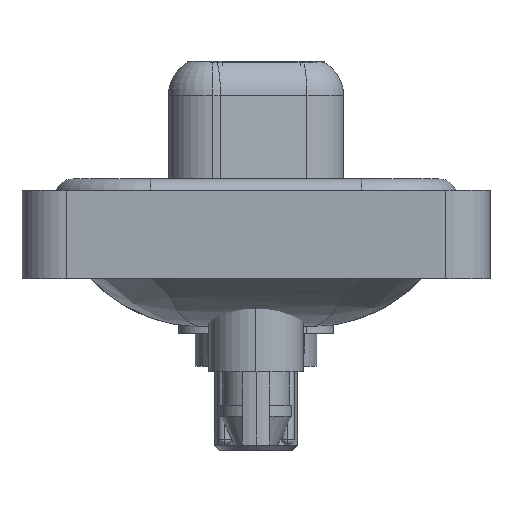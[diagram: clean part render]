
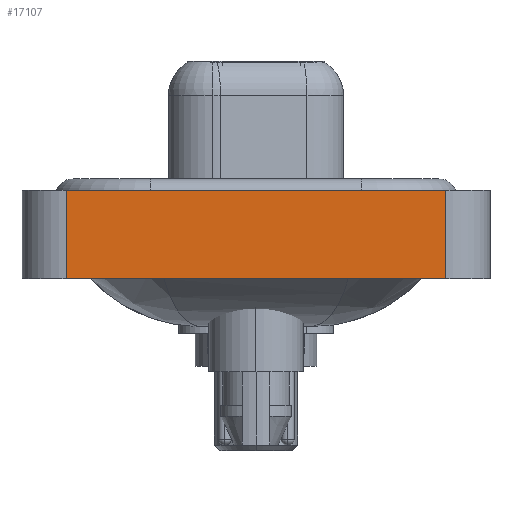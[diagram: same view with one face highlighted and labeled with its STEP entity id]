
A CAD part, left-side view. The second image highlights one B-rep face of the part: STEP entity #17107.
In plain terms, the highlighted planar face has unit normal (-1, 0, 0).
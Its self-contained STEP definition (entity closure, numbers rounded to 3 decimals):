
#50 = LINE ( 'NONE', #14813, #1802 ) ;
#623 = DIRECTION ( 'NONE',  ( -1., 0., 0. ) ) ;
#1398 = ORIENTED_EDGE ( 'NONE', *, *, #5186, .T. ) ;
#1802 = VECTOR ( 'NONE', #6632, 1000. ) ;
#1933 = LINE ( 'NONE', #2036, #13581 ) ;
#2036 = CARTESIAN_POINT ( 'NONE',  ( -7.25, 8.55, -3.6 ) ) ;
#3581 = AXIS2_PLACEMENT_3D ( 'NONE', #15376, #623, #7202 ) ;
#3657 = ORIENTED_EDGE ( 'NONE', *, *, #16149, .F. ) ;
#4423 = VERTEX_POINT ( 'NONE', #12199 ) ;
#4572 = VERTEX_POINT ( 'NONE', #15634 ) ;
#4736 = EDGE_LOOP ( 'NONE', ( #1398, #3657, #8249, #20996 ) ) ;
#5186 = EDGE_CURVE ( 'NONE', #4423, #10924, #50, .T. ) ;
#6632 = DIRECTION ( 'NONE',  ( 0., 0., 1. ) ) ;
#7202 = DIRECTION ( 'NONE',  ( 0., 0., 1. ) ) ;
#8132 = CARTESIAN_POINT ( 'NONE',  ( -7.25, -8.55, -3.6 ) ) ;
#8249 = ORIENTED_EDGE ( 'NONE', *, *, #16529, .F. ) ;
#8818 = FACE_OUTER_BOUND ( 'NONE', #4736, .T. ) ;
#8930 = VERTEX_POINT ( 'NONE', #15590 ) ;
#9345 = VECTOR ( 'NONE', #21254, 1000. ) ;
#9958 = LINE ( 'NONE', #8132, #9345 ) ;
#10924 = VERTEX_POINT ( 'NONE', #14662 ) ;
#11217 = VECTOR ( 'NONE', #11542, 1000. ) ;
#11542 = DIRECTION ( 'NONE',  ( 0., -1., 0. ) ) ;
#12199 = CARTESIAN_POINT ( 'NONE',  ( -7.25, -8.55, -3.6 ) ) ;
#13581 = VECTOR ( 'NONE', #19599, 1000. ) ;
#13585 = LINE ( 'NONE', #20153, #11217 ) ;
#14662 = CARTESIAN_POINT ( 'NONE',  ( -7.25, -8.55, 0.4 ) ) ;
#14813 = CARTESIAN_POINT ( 'NONE',  ( -7.25, -8.55, -3.6 ) ) ;
#15376 = CARTESIAN_POINT ( 'NONE',  ( -7.25, -8.55, -3.6 ) ) ;
#15590 = CARTESIAN_POINT ( 'NONE',  ( -7.25, 8.55, -3.6 ) ) ;
#15594 = PLANE ( 'NONE',  #3581 ) ;
#15634 = CARTESIAN_POINT ( 'NONE',  ( -7.25, 8.55, 0.4 ) ) ;
#16149 = EDGE_CURVE ( 'NONE', #4572, #10924, #13585, .T. ) ;
#16529 = EDGE_CURVE ( 'NONE', #8930, #4572, #1933, .T. ) ;
#17107 = ADVANCED_FACE ( 'NONE', ( #8818 ), #15594, .T. ) ;
#17851 = EDGE_CURVE ( 'NONE', #8930, #4423, #9958, .T. ) ;
#19599 = DIRECTION ( 'NONE',  ( 0., 0., 1. ) ) ;
#20153 = CARTESIAN_POINT ( 'NONE',  ( -7.25, -8.55, 0.4 ) ) ;
#20996 = ORIENTED_EDGE ( 'NONE', *, *, #17851, .T. ) ;
#21254 = DIRECTION ( 'NONE',  ( 0., -1., 0. ) ) ;
